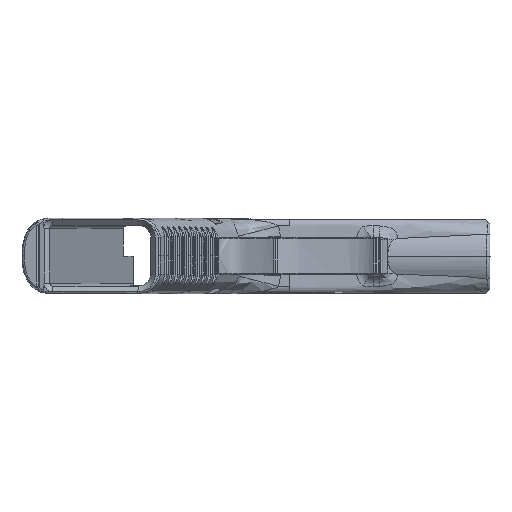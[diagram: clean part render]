
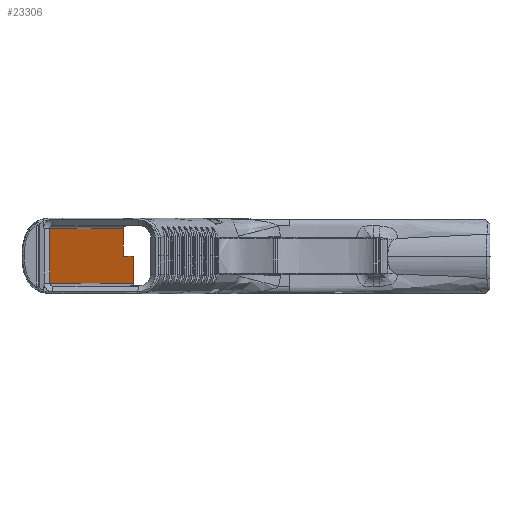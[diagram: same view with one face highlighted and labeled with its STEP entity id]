
A CAD part, top view. The second image highlights one B-rep face of the part: STEP entity #23306.
In plain terms, the highlighted planar face has unit normal (0.951, 0, 0.309).
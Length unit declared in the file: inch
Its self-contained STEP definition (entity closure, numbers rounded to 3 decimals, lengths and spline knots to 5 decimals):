
#2658 = ORIENTED_EDGE ( 'NONE', *, *, #8179, .F. ) ;
#6712 = DIRECTION ( 'NONE',  ( 0., -1., 0. ) ) ;
#7482 = CARTESIAN_POINT ( 'NONE',  ( 2.08094, 0.00002, -3.89598 ) ) ;
#8015 = LINE ( 'NONE', #55776, #24405 ) ;
#8179 = EDGE_CURVE ( 'NONE', #56051, #67780, #12354, .T. ) ;
#12354 = LINE ( 'NONE', #7482, #41129 ) ;
#12704 = EDGE_CURVE ( 'NONE', #65316, #83133, #64587, .T. ) ;
#18296 = DIRECTION ( 'NONE',  ( -0.951, 0., -0.309 ) ) ;
#18586 = CARTESIAN_POINT ( 'NONE',  ( 2.0746, 0., -3.87647 ) ) ;
#23306 = ADVANCED_FACE ( 'NONE', ( #26899 ), #31260, .F. ) ;
#24386 = VERTEX_POINT ( 'NONE', #56367 ) ;
#24405 = VECTOR ( 'NONE', #68955, 39.37008 ) ;
#25614 = ORIENTED_EDGE ( 'NONE', *, *, #32352, .F. ) ;
#26585 = CARTESIAN_POINT ( 'NONE',  ( 2.08094, 0.00006, -3.89598 ) ) ;
#26899 = FACE_OUTER_BOUND ( 'NONE', #82947, .T. ) ;
#28123 = VECTOR ( 'NONE', #69944, 39.37008 ) ;
#30387 = CARTESIAN_POINT ( 'NONE',  ( 2.0746, 0.00006, -3.87647 ) ) ;
#31260 = PLANE ( 'NONE',  #47590 ) ;
#31841 = EDGE_CURVE ( 'NONE', #67780, #39592, #45101, .T. ) ;
#32352 = EDGE_CURVE ( 'NONE', #83133, #24386, #84098, .T. ) ;
#32365 = CARTESIAN_POINT ( 'NONE',  ( 0.94993, 0.37004, -0.41508 ) ) ;
#33077 = CARTESIAN_POINT ( 'NONE',  ( 0.94993, -0.37004, -0.41508 ) ) ;
#33804 = EDGE_CURVE ( 'NONE', #39592, #65316, #8015, .T. ) ;
#33940 = DIRECTION ( 'NONE',  ( -0.309, 0., 0.951 ) ) ;
#36396 = LINE ( 'NONE', #30387, #28123 ) ;
#36871 = VECTOR ( 'NONE', #6712, 39.37008 ) ;
#39592 = VERTEX_POINT ( 'NONE', #33077 ) ;
#41129 = VECTOR ( 'NONE', #76327, 39.37008 ) ;
#45101 = LINE ( 'NONE', #72948, #56360 ) ;
#47590 = AXIS2_PLACEMENT_3D ( 'NONE', #18586, #18296, #70234 ) ;
#48909 = DIRECTION ( 'NONE',  ( 0.309, 0., -0.951 ) ) ;
#53899 = ORIENTED_EDGE ( 'NONE', *, *, #62770, .F. ) ;
#55776 = CARTESIAN_POINT ( 'NONE',  ( 0.94993, 0., -0.41508 ) ) ;
#55812 = CARTESIAN_POINT ( 'NONE',  ( 2.0746, 0.37004, -3.87647 ) ) ;
#56051 = VERTEX_POINT ( 'NONE', #26585 ) ;
#56360 = VECTOR ( 'NONE', #33940, 39.37008 ) ;
#56367 = CARTESIAN_POINT ( 'NONE',  ( 1.94663, 0.00006, -3.4826 ) ) ;
#60468 = CARTESIAN_POINT ( 'NONE',  ( 2.08094, -0.37004, -3.89598 ) ) ;
#62770 = EDGE_CURVE ( 'NONE', #24386, #56051, #36396, .T. ) ;
#64587 = LINE ( 'NONE', #55812, #67704 ) ;
#64952 = ORIENTED_EDGE ( 'NONE', *, *, #33804, .F. ) ;
#65316 = VERTEX_POINT ( 'NONE', #32365 ) ;
#67704 = VECTOR ( 'NONE', #48909, 39.37008 ) ;
#67780 = VERTEX_POINT ( 'NONE', #60468 ) ;
#68955 = DIRECTION ( 'NONE',  ( 0., 1., 0. ) ) ;
#69944 = DIRECTION ( 'NONE',  ( 0.309, 0., -0.951 ) ) ;
#70228 = ORIENTED_EDGE ( 'NONE', *, *, #31841, .F. ) ;
#70234 = DIRECTION ( 'NONE',  ( -0.309, 0., 0.951 ) ) ;
#72948 = CARTESIAN_POINT ( 'NONE',  ( 2.0746, -0.37004, -3.87647 ) ) ;
#76327 = DIRECTION ( 'NONE',  ( 0., -1., 0. ) ) ;
#79020 = CARTESIAN_POINT ( 'NONE',  ( 1.94663, 0., -3.4826 ) ) ;
#79306 = ORIENTED_EDGE ( 'NONE', *, *, #12704, .F. ) ;
#82314 = CARTESIAN_POINT ( 'NONE',  ( 1.94663, 0.37004, -3.4826 ) ) ;
#82947 = EDGE_LOOP ( 'NONE', ( #25614, #79306, #64952, #70228, #2658, #53899 ) ) ;
#83133 = VERTEX_POINT ( 'NONE', #82314 ) ;
#84098 = LINE ( 'NONE', #79020, #36871 ) ;
